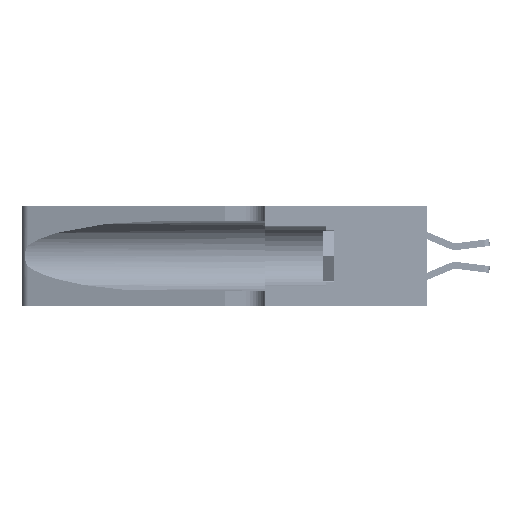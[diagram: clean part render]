
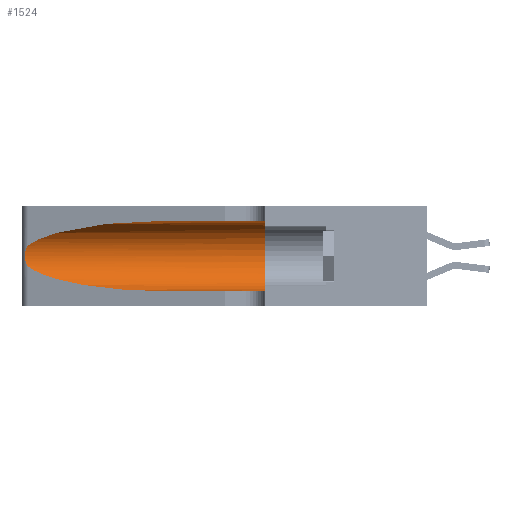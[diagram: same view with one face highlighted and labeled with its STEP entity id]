
A CAD part, left-side view. The second image highlights one B-rep face of the part: STEP entity #1524.
In plain terms, the highlighted cylindrical face has radius 3.308 mm (diameter 6.617 mm), a partial arc.
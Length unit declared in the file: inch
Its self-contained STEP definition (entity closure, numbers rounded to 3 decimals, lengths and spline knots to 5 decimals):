
#493 = EDGE_CURVE ( 'NONE', #3990, #17581, #6134, .T. ) ;
#874 = CARTESIAN_POINT ( 'NONE',  ( 0.1305, 0.72297, 0.05475 ) ) ;
#1396 = CARTESIAN_POINT ( 'NONE',  ( 0.26075, 1.23896, 0.178 ) ) ;
#1524 = ADVANCED_FACE ( 'NONE', ( #11763 ), #18856, .F. ) ;
#2006 = VERTEX_POINT ( 'NONE', #874 ) ;
#2436 = CARTESIAN_POINT ( 'NONE',  ( 0.1305, 0.72297, 0.31525 ) ) ;
#2714 = CARTESIAN_POINT ( 'NONE',  ( 0.25487, 1.22718, 0.22369 ) ) ;
#3990 = VERTEX_POINT ( 'NONE', #12347 ) ;
#4525 = CARTESIAN_POINT ( 'NONE',  ( 0.25856, 1.23593, 0.16098 ) ) ;
#4565 = VERTEX_POINT ( 'NONE', #17880 ) ;
#4577 = LINE ( 'NONE', #14011, #18850 ) ;
#5321 = AXIS2_PLACEMENT_3D ( 'NONE', #29145, #13639, #11021 ) ;
#6133 = EDGE_LOOP ( 'NONE', ( #37190, #22951, #23442, #38115, #32016, #8330 ) ) ;
#6134 =( BOUNDED_CURVE ( )  B_SPLINE_CURVE ( 3, ( #2436, #16335, #20900, #2714 ),
 .UNSPECIFIED., .F., .F. ) 
 B_SPLINE_CURVE_WITH_KNOTS ( ( 4, 4 ),
 ( 1.5708, 2.84003 ),
 .UNSPECIFIED. ) 
 CURVE ( )  GEOMETRIC_REPRESENTATION_ITEM ( )  RATIONAL_B_SPLINE_CURVE ( ( 1., 0.87, 0.87, 1. ) ) 
 REPRESENTATION_ITEM ( '' )  );
#7476 = CARTESIAN_POINT ( 'NONE',  ( 0.25487, 1.22718, 0.22369 ) ) ;
#7614 = CARTESIAN_POINT ( 'NONE',  ( 0.25639, 1.23186, 0.15144 ) ) ;
#8263 = CARTESIAN_POINT ( 'NONE',  ( 0.1305, 0.35, 0.31525 ) ) ;
#8330 = ORIENTED_EDGE ( 'NONE', *, *, #32283, .F. ) ;
#10700 = CARTESIAN_POINT ( 'NONE',  ( 0.25487, 1.22718, 0.14631 ) ) ;
#11021 = DIRECTION ( 'NONE',  ( 0., 0., -1. ) ) ;
#11763 = FACE_OUTER_BOUND ( 'NONE', #6133, .T. ) ;
#11990 = LINE ( 'NONE', #13979, #21942 ) ;
#12347 = CARTESIAN_POINT ( 'NONE',  ( 0.1305, 0.72297, 0.31525 ) ) ;
#13187 = EDGE_CURVE ( 'NONE', #22827, #4565, #33990, .T. ) ;
#13569 = CARTESIAN_POINT ( 'NONE',  ( 0.25639, 1.23184, 0.21858 ) ) ;
#13639 = DIRECTION ( 'NONE',  ( 0., -1., 0. ) ) ;
#13979 = CARTESIAN_POINT ( 'NONE',  ( 0.1305, 1.61858, 0.31525 ) ) ;
#14011 = CARTESIAN_POINT ( 'NONE',  ( 0.1305, 1.61858, 0.05475 ) ) ;
#14864 = EDGE_CURVE ( 'NONE', #27827, #2006, #28463, .T. ) ;
#15763 = CARTESIAN_POINT ( 'NONE',  ( 0.1305, 0.72297, 0.05475 ) ) ;
#16335 = CARTESIAN_POINT ( 'NONE',  ( 0.18966, 0.96281, 0.31525 ) ) ;
#16626 = CARTESIAN_POINT ( 'NONE',  ( 0.25854, 1.2359, 0.20912 ) ) ;
#16951 = CARTESIAN_POINT ( 'NONE',  ( 0.1305, 0.35, 0.185 ) ) ;
#17190 = DIRECTION ( 'NONE',  ( 0., -1., 0. ) ) ;
#17581 = VERTEX_POINT ( 'NONE', #29183 ) ;
#17880 = CARTESIAN_POINT ( 'NONE',  ( 0.1305, 0.35, 0.05475 ) ) ;
#18850 = VECTOR ( 'NONE', #17190, 39.37008 ) ;
#18856 = CYLINDRICAL_SURFACE ( 'NONE', #5321, 0.13025 ) ;
#19702 = CARTESIAN_POINT ( 'NONE',  ( 0.26075, 1.23896, 0.19203 ) ) ;
#20027 = DIRECTION ( 'NONE',  ( 0., 0., 1. ) ) ;
#20900 = CARTESIAN_POINT ( 'NONE',  ( 0.2373, 1.15595, 0.28018 ) ) ;
#21942 = VECTOR ( 'NONE', #32120, 39.37008 ) ;
#22741 = CARTESIAN_POINT ( 'NONE',  ( 0.26017, 1.23833, 0.17102 ) ) ;
#22827 = VERTEX_POINT ( 'NONE', #8263 ) ;
#22951 = ORIENTED_EDGE ( 'NONE', *, *, #27705, .T. ) ;
#23442 = ORIENTED_EDGE ( 'NONE', *, *, #14864, .T. ) ;
#24174 = EDGE_CURVE ( 'NONE', #2006, #4565, #4577, .T. ) ;
#25782 = CARTESIAN_POINT ( 'NONE',  ( 0.25789, 1.23486, 0.15765 ) ) ;
#26168 = CARTESIAN_POINT ( 'NONE',  ( 0.25487, 1.22718, 0.14631 ) ) ;
#27705 = EDGE_CURVE ( 'NONE', #17581, #27827, #35657, .T. ) ;
#27827 = VERTEX_POINT ( 'NONE', #26168 ) ;
#28463 =( BOUNDED_CURVE ( )  B_SPLINE_CURVE ( 3, ( #30733, #36697, #33924, #15763 ),
 .UNSPECIFIED., .F., .F. ) 
 B_SPLINE_CURVE_WITH_KNOTS ( ( 4, 4 ),
 ( 3.44316, 4.71239 ),
 .UNSPECIFIED. ) 
 CURVE ( )  GEOMETRIC_REPRESENTATION_ITEM ( )  RATIONAL_B_SPLINE_CURVE ( ( 1., 0.87, 0.87, 1. ) ) 
 REPRESENTATION_ITEM ( '' )  );
#28817 = CARTESIAN_POINT ( 'NONE',  ( 0.25555, 1.22993, 0.14849 ) ) ;
#29145 = CARTESIAN_POINT ( 'NONE',  ( 0.1305, 1.61858, 0.185 ) ) ;
#29183 = CARTESIAN_POINT ( 'NONE',  ( 0.25487, 1.22718, 0.22369 ) ) ;
#30733 = CARTESIAN_POINT ( 'NONE',  ( 0.25487, 1.22718, 0.14631 ) ) ;
#31548 = AXIS2_PLACEMENT_3D ( 'NONE', #16951, #38117, #20027 ) ;
#32016 = ORIENTED_EDGE ( 'NONE', *, *, #13187, .F. ) ;
#32120 = DIRECTION ( 'NONE',  ( 0., -1., 0. ) ) ;
#32283 = EDGE_CURVE ( 'NONE', #3990, #22827, #11990, .T. ) ;
#33924 = CARTESIAN_POINT ( 'NONE',  ( 0.18966, 0.96281, 0.05475 ) ) ;
#33990 = CIRCLE ( 'NONE', #31548, 0.13025 ) ;
#34763 = CARTESIAN_POINT ( 'NONE',  ( 0.25787, 1.23484, 0.2124 ) ) ;
#35657 = B_SPLINE_CURVE_WITH_KNOTS ( 'NONE', 3,
 ( #7476, #37662, #13569, #34763, #16626, #37789, #19702, #1396, #22741, #4525, #25782, #7614, #28817, #10700 ),
 .UNSPECIFIED., .F., .F.,
 ( 4, 2, 2, 2, 2, 2, 4 ),
 ( 0., 0.00027, 0.00053, 0.00107, 0.0016, 0.00187, 0.00214 ),
 .UNSPECIFIED. ) ;
#36697 = CARTESIAN_POINT ( 'NONE',  ( 0.2373, 1.15595, 0.08982 ) ) ;
#37190 = ORIENTED_EDGE ( 'NONE', *, *, #493, .T. ) ;
#37662 = CARTESIAN_POINT ( 'NONE',  ( 0.25555, 1.22994, 0.2215 ) ) ;
#37789 = CARTESIAN_POINT ( 'NONE',  ( 0.26018, 1.23835, 0.19895 ) ) ;
#38115 = ORIENTED_EDGE ( 'NONE', *, *, #24174, .T. ) ;
#38117 = DIRECTION ( 'NONE',  ( 0., 1., 0. ) ) ;
